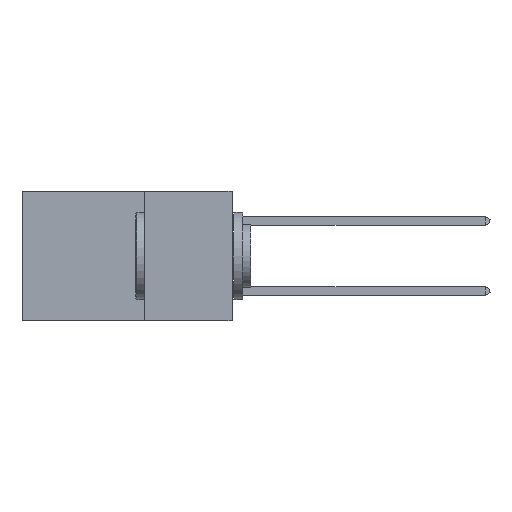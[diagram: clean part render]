
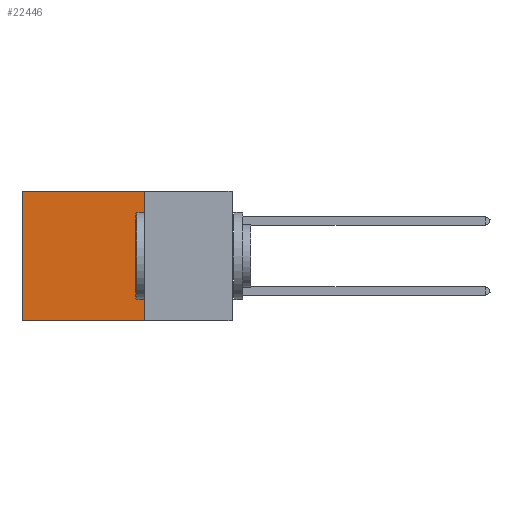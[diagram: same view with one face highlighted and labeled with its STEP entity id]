
A CAD part, left-side view. The second image highlights one B-rep face of the part: STEP entity #22446.
In plain terms, the highlighted planar face has unit normal (-1, 0, 0).
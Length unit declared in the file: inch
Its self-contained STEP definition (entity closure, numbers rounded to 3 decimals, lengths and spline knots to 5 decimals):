
#749 = EDGE_LOOP ( 'NONE', ( #4314, #20496, #15513, #23200 ) ) ;
#1605 = DIRECTION ( 'NONE',  ( 0., 0., -1. ) ) ;
#3803 = FACE_OUTER_BOUND ( 'NONE', #749, .T. ) ;
#4314 = ORIENTED_EDGE ( 'NONE', *, *, #40669, .T. ) ;
#5945 = DIRECTION ( 'NONE',  ( 0., 1., 0. ) ) ;
#5970 = AXIS2_PLACEMENT_3D ( 'NONE', #15085, #22001, #1605 ) ;
#7674 = EDGE_CURVE ( 'NONE', #8144, #43442, #9307, .T. ) ;
#8144 = VERTEX_POINT ( 'NONE', #15223 ) ;
#8153 = VERTEX_POINT ( 'NONE', #18553 ) ;
#9122 = VERTEX_POINT ( 'NONE', #41369 ) ;
#9307 = LINE ( 'NONE', #37517, #17944 ) ;
#10287 = DIRECTION ( 'NONE',  ( 0., 0., -1. ) ) ;
#11074 = EDGE_CURVE ( 'NONE', #8144, #8153, #37238, .T. ) ;
#13269 = DIRECTION ( 'NONE',  ( 0., 0., -1. ) ) ;
#13747 = CARTESIAN_POINT ( 'NONE',  ( 0.2875, 0.6, 0. ) ) ;
#15085 = CARTESIAN_POINT ( 'NONE',  ( 0.2875, 0.25, 0. ) ) ;
#15223 = CARTESIAN_POINT ( 'NONE',  ( 0.2875, 0.25, 0. ) ) ;
#15513 = ORIENTED_EDGE ( 'NONE', *, *, #11074, .F. ) ;
#17727 = VECTOR ( 'NONE', #42722, 39.37008 ) ;
#17944 = VECTOR ( 'NONE', #5945, 39.37008 ) ;
#18553 = CARTESIAN_POINT ( 'NONE',  ( 0.2875, 0.25, -0.37 ) ) ;
#18707 = CARTESIAN_POINT ( 'NONE',  ( 0.2875, 0.25, -0.37 ) ) ;
#20496 = ORIENTED_EDGE ( 'NONE', *, *, #37595, .F. ) ;
#22001 = DIRECTION ( 'NONE',  ( 1., 0., 0. ) ) ;
#22446 = ADVANCED_FACE ( 'NONE', ( #3803 ), #29218, .F. ) ;
#23200 = ORIENTED_EDGE ( 'NONE', *, *, #7674, .T. ) ;
#26046 = CARTESIAN_POINT ( 'NONE',  ( 0.2875, 0.6, 0. ) ) ;
#26857 = LINE ( 'NONE', #18707, #17727 ) ;
#28056 = VECTOR ( 'NONE', #13269, 39.37008 ) ;
#29218 = PLANE ( 'NONE',  #5970 ) ;
#33886 = CARTESIAN_POINT ( 'NONE',  ( 0.2875, 0.25, 0. ) ) ;
#36659 = VECTOR ( 'NONE', #10287, 39.37008 ) ;
#37238 = LINE ( 'NONE', #33886, #28056 ) ;
#37517 = CARTESIAN_POINT ( 'NONE',  ( 0.2875, 0.25, 0. ) ) ;
#37595 = EDGE_CURVE ( 'NONE', #8153, #9122, #26857, .T. ) ;
#40669 = EDGE_CURVE ( 'NONE', #43442, #9122, #42524, .T. ) ;
#41369 = CARTESIAN_POINT ( 'NONE',  ( 0.2875, 0.6, -0.37 ) ) ;
#42524 = LINE ( 'NONE', #13747, #36659 ) ;
#42722 = DIRECTION ( 'NONE',  ( 0., 1., 0. ) ) ;
#43442 = VERTEX_POINT ( 'NONE', #26046 ) ;
